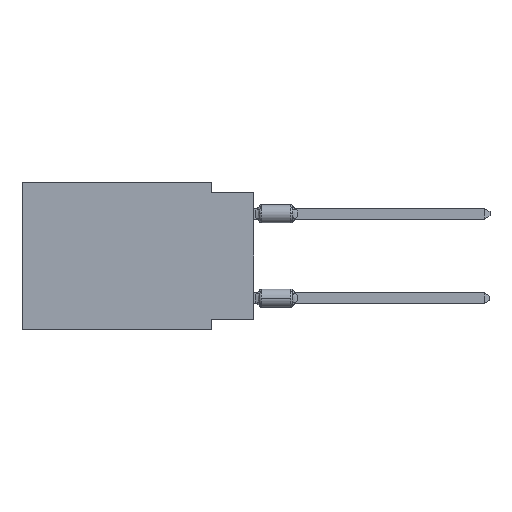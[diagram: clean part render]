
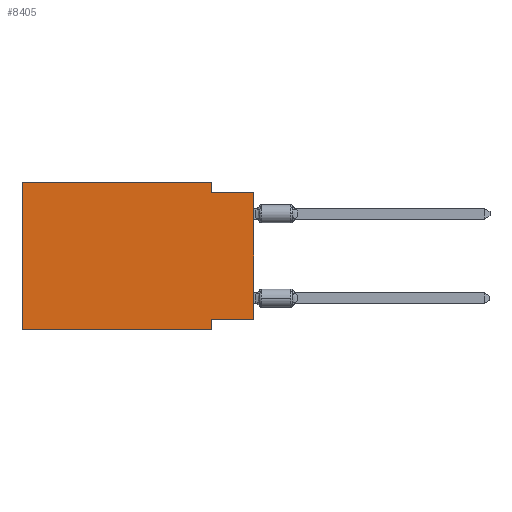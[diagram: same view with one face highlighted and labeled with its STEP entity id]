
A CAD part, left-side view. The second image highlights one B-rep face of the part: STEP entity #8405.
In plain terms, the highlighted planar face has unit normal (-1, 0, 0).
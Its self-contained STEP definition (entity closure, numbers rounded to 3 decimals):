
#165 = VECTOR ( 'NONE', #13366, 1000. ) ;
#450 = ORIENTED_EDGE ( 'NONE', *, *, #8725, .F. ) ;
#513 = CARTESIAN_POINT ( 'NONE',  ( 0., 2.54, -8.89 ) ) ;
#524 = VERTEX_POINT ( 'NONE', #2728 ) ;
#740 = LINE ( 'NONE', #7770, #165 ) ;
#1379 = CARTESIAN_POINT ( 'NONE',  ( 0., 13.97, 0. ) ) ;
#1447 = DIRECTION ( 'NONE',  ( 0., 0., -1. ) ) ;
#1649 = AXIS2_PLACEMENT_3D ( 'NONE', #8552, #13881, #6836 ) ;
#1760 = ORIENTED_EDGE ( 'NONE', *, *, #12888, .F. ) ;
#1793 = DIRECTION ( 'NONE',  ( 0., 0., 1. ) ) ;
#2157 = CARTESIAN_POINT ( 'NONE',  ( 0., 0., 0. ) ) ;
#2436 = CARTESIAN_POINT ( 'NONE',  ( 0., 0., -8.255 ) ) ;
#2728 = CARTESIAN_POINT ( 'NONE',  ( 0., 13.97, -8.89 ) ) ;
#3180 = ORIENTED_EDGE ( 'NONE', *, *, #12448, .F. ) ;
#3428 = VECTOR ( 'NONE', #14762, 1000. ) ;
#3600 = LINE ( 'NONE', #14669, #3428 ) ;
#3717 = CARTESIAN_POINT ( 'NONE',  ( 0., 0., -0.635 ) ) ;
#4360 = VERTEX_POINT ( 'NONE', #15742 ) ;
#4785 = VERTEX_POINT ( 'NONE', #513 ) ;
#4901 = LINE ( 'NONE', #2157, #6636 ) ;
#4954 = VECTOR ( 'NONE', #15269, 1000. ) ;
#5645 = VERTEX_POINT ( 'NONE', #8599 ) ;
#5752 = CARTESIAN_POINT ( 'NONE',  ( 0., 2.54, -0.635 ) ) ;
#6058 = LINE ( 'NONE', #10254, #14424 ) ;
#6365 = LINE ( 'NONE', #3717, #14273 ) ;
#6467 = ORIENTED_EDGE ( 'NONE', *, *, #14937, .T. ) ;
#6636 = VECTOR ( 'NONE', #1793, 1000. ) ;
#6836 = DIRECTION ( 'NONE',  ( 0., 0., -1. ) ) ;
#6889 = VERTEX_POINT ( 'NONE', #7476 ) ;
#7241 = EDGE_CURVE ( 'NONE', #16101, #9810, #11041, .T. ) ;
#7476 = CARTESIAN_POINT ( 'NONE',  ( 0., 0., -8.255 ) ) ;
#7770 = CARTESIAN_POINT ( 'NONE',  ( 0., 13.97, -8.89 ) ) ;
#8313 = ORIENTED_EDGE ( 'NONE', *, *, #15717, .T. ) ;
#8325 = VECTOR ( 'NONE', #1447, 1000. ) ;
#8380 = CARTESIAN_POINT ( 'NONE',  ( 0., 2.54, 0. ) ) ;
#8405 = ADVANCED_FACE ( 'NONE', ( #13794 ), #16711, .F. ) ;
#8552 = CARTESIAN_POINT ( 'NONE',  ( 0., 13.97, 0. ) ) ;
#8599 = CARTESIAN_POINT ( 'NONE',  ( 0., 13.97, 0. ) ) ;
#8725 = EDGE_CURVE ( 'NONE', #6889, #4360, #10846, .T. ) ;
#9121 = EDGE_CURVE ( 'NONE', #4360, #4785, #3600, .T. ) ;
#9263 = VECTOR ( 'NONE', #11955, 1000. ) ;
#9810 = VERTEX_POINT ( 'NONE', #5752 ) ;
#10254 = CARTESIAN_POINT ( 'NONE',  ( 0., 13.97, 0. ) ) ;
#10507 = ORIENTED_EDGE ( 'NONE', *, *, #7241, .F. ) ;
#10846 = LINE ( 'NONE', #2436, #9263 ) ;
#11041 = LINE ( 'NONE', #8380, #8325 ) ;
#11440 = CARTESIAN_POINT ( 'NONE',  ( 0., 0., -0.635 ) ) ;
#11955 = DIRECTION ( 'NONE',  ( 0., 1., 0. ) ) ;
#12237 = ORIENTED_EDGE ( 'NONE', *, *, #9121, .F. ) ;
#12448 = EDGE_CURVE ( 'NONE', #9810, #15683, #6365, .T. ) ;
#12801 = LINE ( 'NONE', #1379, #4954 ) ;
#12888 = EDGE_CURVE ( 'NONE', #5645, #16101, #12801, .T. ) ;
#13366 = DIRECTION ( 'NONE',  ( 0., -1., 0. ) ) ;
#13794 = FACE_OUTER_BOUND ( 'NONE', #17075, .T. ) ;
#13881 = DIRECTION ( 'NONE',  ( 1., 0., 0. ) ) ;
#14273 = VECTOR ( 'NONE', #17710, 1000. ) ;
#14424 = VECTOR ( 'NONE', #15923, 1000. ) ;
#14434 = CARTESIAN_POINT ( 'NONE',  ( 0., 2.54, 0. ) ) ;
#14669 = CARTESIAN_POINT ( 'NONE',  ( 0., 2.54, -8.89 ) ) ;
#14762 = DIRECTION ( 'NONE',  ( 0., 0., -1. ) ) ;
#14937 = EDGE_CURVE ( 'NONE', #6889, #15683, #4901, .T. ) ;
#15269 = DIRECTION ( 'NONE',  ( 0., -1., 0. ) ) ;
#15683 = VERTEX_POINT ( 'NONE', #11440 ) ;
#15717 = EDGE_CURVE ( 'NONE', #524, #4785, #740, .T. ) ;
#15742 = CARTESIAN_POINT ( 'NONE',  ( 0., 2.54, -8.255 ) ) ;
#15923 = DIRECTION ( 'NONE',  ( 0., 0., 1. ) ) ;
#16101 = VERTEX_POINT ( 'NONE', #14434 ) ;
#16711 = PLANE ( 'NONE',  #1649 ) ;
#16861 = EDGE_CURVE ( 'NONE', #524, #5645, #6058, .T. ) ;
#17075 = EDGE_LOOP ( 'NONE', ( #6467, #3180, #10507, #1760, #17415, #8313, #12237, #450 ) ) ;
#17415 = ORIENTED_EDGE ( 'NONE', *, *, #16861, .F. ) ;
#17710 = DIRECTION ( 'NONE',  ( 0., -1., 0. ) ) ;
